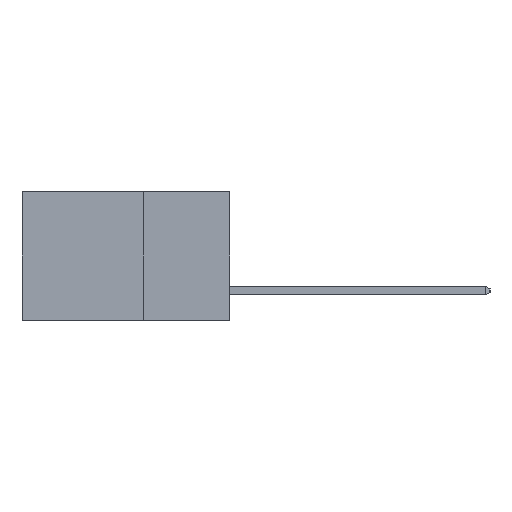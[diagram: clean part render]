
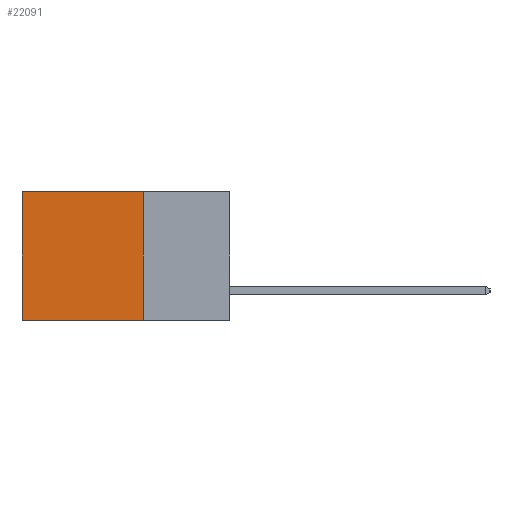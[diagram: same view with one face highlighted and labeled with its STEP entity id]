
A CAD part, left-side view. The second image highlights one B-rep face of the part: STEP entity #22091.
In plain terms, the highlighted planar face has unit normal (-1, 0, 0).
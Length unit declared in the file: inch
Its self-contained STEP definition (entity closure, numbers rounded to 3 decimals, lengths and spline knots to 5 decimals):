
#425 = DIRECTION ( 'NONE',  ( 0., 0., -1. ) ) ;
#430 = CARTESIAN_POINT ( 'NONE',  ( 0.298, 0.6, 0. ) ) ;
#1464 = ORIENTED_EDGE ( 'NONE', *, *, #17391, .F. ) ;
#1548 = CARTESIAN_POINT ( 'NONE',  ( 0.298, 0.6, -0.37 ) ) ;
#1986 = DIRECTION ( 'NONE',  ( 0., 1., 0. ) ) ;
#2303 = CARTESIAN_POINT ( 'NONE',  ( 0.298, 0.25, 0. ) ) ;
#2307 = VECTOR ( 'NONE', #3130, 39.37008 ) ;
#3130 = DIRECTION ( 'NONE',  ( 0., 0., -1. ) ) ;
#3757 = ORIENTED_EDGE ( 'NONE', *, *, #5161, .T. ) ;
#4073 = DIRECTION ( 'NONE',  ( 0., 0., -1. ) ) ;
#4767 = VECTOR ( 'NONE', #1986, 39.37008 ) ;
#4925 = LINE ( 'NONE', #430, #18880 ) ;
#5161 = EDGE_CURVE ( 'NONE', #19086, #13782, #4925, .T. ) ;
#5755 = CARTESIAN_POINT ( 'NONE',  ( 0.298, 0.6, 0. ) ) ;
#5794 = ORIENTED_EDGE ( 'NONE', *, *, #13743, .F. ) ;
#5919 = EDGE_LOOP ( 'NONE', ( #3757, #1464, #5794, #14562 ) ) ;
#6900 = LINE ( 'NONE', #14467, #15716 ) ;
#11638 = FACE_OUTER_BOUND ( 'NONE', #5919, .T. ) ;
#11854 = CARTESIAN_POINT ( 'NONE',  ( 0.298, 0.25, 0. ) ) ;
#12459 = CARTESIAN_POINT ( 'NONE',  ( 0.298, 0.25, 0. ) ) ;
#13743 = EDGE_CURVE ( 'NONE', #21604, #15500, #15776, .T. ) ;
#13782 = VERTEX_POINT ( 'NONE', #1548 ) ;
#14467 = CARTESIAN_POINT ( 'NONE',  ( 0.298, 0.25, -0.37 ) ) ;
#14562 = ORIENTED_EDGE ( 'NONE', *, *, #17242, .T. ) ;
#14563 = DIRECTION ( 'NONE',  ( 1., 0., 0. ) ) ;
#15500 = VERTEX_POINT ( 'NONE', #19552 ) ;
#15716 = VECTOR ( 'NONE', #17980, 39.37008 ) ;
#15776 = LINE ( 'NONE', #11854, #2307 ) ;
#17242 = EDGE_CURVE ( 'NONE', #21604, #19086, #19787, .T. ) ;
#17391 = EDGE_CURVE ( 'NONE', #15500, #13782, #6900, .T. ) ;
#17980 = DIRECTION ( 'NONE',  ( 0., 1., 0. ) ) ;
#18239 = CARTESIAN_POINT ( 'NONE',  ( 0.298, 0.25, 0. ) ) ;
#18880 = VECTOR ( 'NONE', #425, 39.37008 ) ;
#19086 = VERTEX_POINT ( 'NONE', #5755 ) ;
#19552 = CARTESIAN_POINT ( 'NONE',  ( 0.298, 0.25, -0.37 ) ) ;
#19787 = LINE ( 'NONE', #12459, #4767 ) ;
#21136 = PLANE ( 'NONE',  #22521 ) ;
#21604 = VERTEX_POINT ( 'NONE', #18239 ) ;
#22091 = ADVANCED_FACE ( 'NONE', ( #11638 ), #21136, .F. ) ;
#22521 = AXIS2_PLACEMENT_3D ( 'NONE', #2303, #14563, #4073 ) ;
